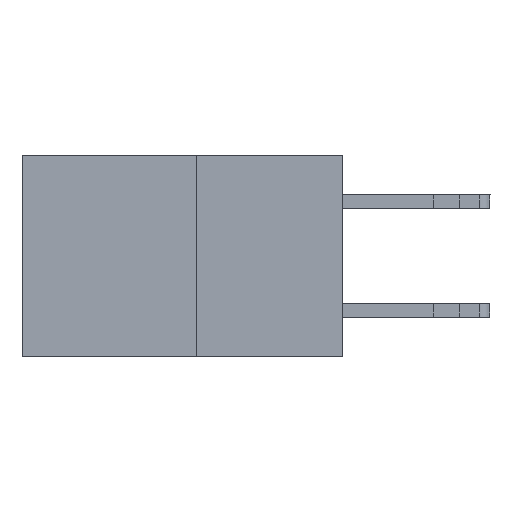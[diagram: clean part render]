
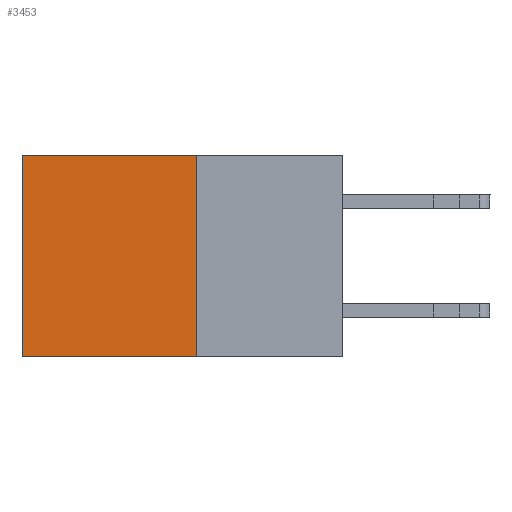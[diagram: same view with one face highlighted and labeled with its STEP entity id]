
A CAD part, left-side view. The second image highlights one B-rep face of the part: STEP entity #3453.
In plain terms, the highlighted planar face has unit normal (-1, 0, 0).
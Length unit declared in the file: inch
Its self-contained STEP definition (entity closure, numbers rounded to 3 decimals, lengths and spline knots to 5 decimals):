
#731 = VERTEX_POINT ( 'NONE', #4017 ) ;
#2088 = LINE ( 'NONE', #10404, #21106 ) ;
#3453 = ADVANCED_FACE ( 'NONE', ( #16161 ), #20825, .F. ) ;
#3799 = ORIENTED_EDGE ( 'NONE', *, *, #25221, .F. ) ;
#4017 = CARTESIAN_POINT ( 'NONE',  ( 0.277, 0.59, -0.37 ) ) ;
#4511 = LINE ( 'NONE', #6649, #15768 ) ;
#5309 = EDGE_LOOP ( 'NONE', ( #6183, #3799, #25498, #10511 ) ) ;
#5452 = VECTOR ( 'NONE', #21791, 39.37008 ) ;
#6130 = CARTESIAN_POINT ( 'NONE',  ( 0.277, 0.27, -0.37 ) ) ;
#6183 = ORIENTED_EDGE ( 'NONE', *, *, #10666, .T. ) ;
#6649 = CARTESIAN_POINT ( 'NONE',  ( 0.277, 0.59, -0.37 ) ) ;
#6792 = VERTEX_POINT ( 'NONE', #10937 ) ;
#9974 = AXIS2_PLACEMENT_3D ( 'NONE', #6130, #12287, #18297 ) ;
#10404 = CARTESIAN_POINT ( 'NONE',  ( 0.277, 0.27, 0. ) ) ;
#10511 = ORIENTED_EDGE ( 'NONE', *, *, #12692, .T. ) ;
#10666 = EDGE_CURVE ( 'NONE', #16083, #731, #4511, .T. ) ;
#10937 = CARTESIAN_POINT ( 'NONE',  ( 0.277, 0.27, -0.37 ) ) ;
#12287 = DIRECTION ( 'NONE',  ( 1., 0., 0. ) ) ;
#12692 = EDGE_CURVE ( 'NONE', #13442, #16083, #2088, .T. ) ;
#13442 = VERTEX_POINT ( 'NONE', #14101 ) ;
#14101 = CARTESIAN_POINT ( 'NONE',  ( 0.277, 0.27, 0. ) ) ;
#14950 = EDGE_CURVE ( 'NONE', #13442, #6792, #23661, .T. ) ;
#15768 = VECTOR ( 'NONE', #22920, 39.37008 ) ;
#16083 = VERTEX_POINT ( 'NONE', #21673 ) ;
#16161 = FACE_OUTER_BOUND ( 'NONE', #5309, .T. ) ;
#17180 = VECTOR ( 'NONE', #17569, 39.37008 ) ;
#17569 = DIRECTION ( 'NONE',  ( 0., 1., 0. ) ) ;
#17946 = CARTESIAN_POINT ( 'NONE',  ( 0.277, 0.27, -0.37 ) ) ;
#18297 = DIRECTION ( 'NONE',  ( 0., 0., -1. ) ) ;
#18559 = DIRECTION ( 'NONE',  ( 0., 1., 0. ) ) ;
#19083 = LINE ( 'NONE', #21797, #17180 ) ;
#20825 = PLANE ( 'NONE',  #9974 ) ;
#21106 = VECTOR ( 'NONE', #18559, 39.37008 ) ;
#21673 = CARTESIAN_POINT ( 'NONE',  ( 0.277, 0.59, 0. ) ) ;
#21791 = DIRECTION ( 'NONE',  ( 0., 0., -1. ) ) ;
#21797 = CARTESIAN_POINT ( 'NONE',  ( 0.277, 0.27, -0.37 ) ) ;
#22920 = DIRECTION ( 'NONE',  ( 0., 0., -1. ) ) ;
#23661 = LINE ( 'NONE', #17946, #5452 ) ;
#25221 = EDGE_CURVE ( 'NONE', #6792, #731, #19083, .T. ) ;
#25498 = ORIENTED_EDGE ( 'NONE', *, *, #14950, .F. ) ;
